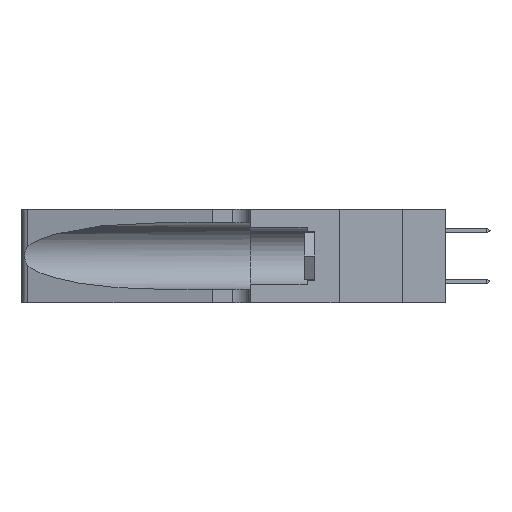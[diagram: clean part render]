
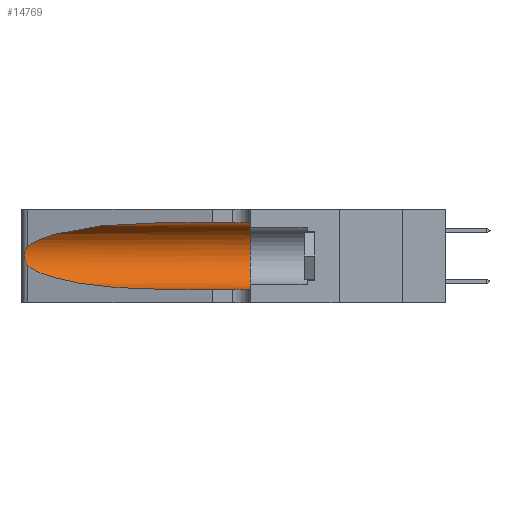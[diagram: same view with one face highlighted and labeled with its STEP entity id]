
A CAD part, left-side view. The second image highlights one B-rep face of the part: STEP entity #14769.
In plain terms, the highlighted cylindrical face has radius 3.308 mm (diameter 6.617 mm), a partial arc.
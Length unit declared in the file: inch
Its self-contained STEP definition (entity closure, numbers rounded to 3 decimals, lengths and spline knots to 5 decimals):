
#147 = CARTESIAN_POINT ( 'NONE',  ( 0.1305, 0.35, 0.185 ) ) ;
#178 = CARTESIAN_POINT ( 'NONE',  ( 0.25487, 1.22718, 0.14631 ) ) ;
#475 = CARTESIAN_POINT ( 'NONE',  ( 0.25555, 1.22994, 0.2215 ) ) ;
#570 = CARTESIAN_POINT ( 'NONE',  ( 0.25639, 1.23186, 0.15144 ) ) ;
#1190 = DIRECTION ( 'NONE',  ( 0., -1., 0. ) ) ;
#1701 = ORIENTED_EDGE ( 'NONE', *, *, #25862, .T. ) ;
#2406 = CARTESIAN_POINT ( 'NONE',  ( 0.2373, 1.15595, 0.08982 ) ) ;
#2423 = CARTESIAN_POINT ( 'NONE',  ( 0.1305, 0.35, 0.31525 ) ) ;
#2620 = DIRECTION ( 'NONE',  ( 0., 0., 1. ) ) ;
#3052 = CARTESIAN_POINT ( 'NONE',  ( 0.25487, 1.22718, 0.14631 ) ) ;
#3651 = CARTESIAN_POINT ( 'NONE',  ( 0.1305, 0.35, 0.05475 ) ) ;
#5392 = CARTESIAN_POINT ( 'NONE',  ( 0.25639, 1.23184, 0.21858 ) ) ;
#5688 = VECTOR ( 'NONE', #16708, 39.37008 ) ;
#5945 = CARTESIAN_POINT ( 'NONE',  ( 0.2373, 1.15595, 0.28018 ) ) ;
#5985 = DIRECTION ( 'NONE',  ( 0., 0., -1. ) ) ;
#6005 = CARTESIAN_POINT ( 'NONE',  ( 0.1305, 0.72297, 0.31525 ) ) ;
#6544 = EDGE_CURVE ( 'NONE', #20470, #12435, #19290, .T. ) ;
#6942 = ORIENTED_EDGE ( 'NONE', *, *, #23204, .T. ) ;
#7333 = CARTESIAN_POINT ( 'NONE',  ( 0.1305, 0.72297, 0.05475 ) ) ;
#7843 = ORIENTED_EDGE ( 'NONE', *, *, #6544, .T. ) ;
#7873 = CARTESIAN_POINT ( 'NONE',  ( 0.25854, 1.2359, 0.20912 ) ) ;
#9403 = ORIENTED_EDGE ( 'NONE', *, *, #28127, .T. ) ;
#9880 = CARTESIAN_POINT ( 'NONE',  ( 0.1305, 0.72297, 0.05475 ) ) ;
#10054 = VERTEX_POINT ( 'NONE', #2423 ) ;
#10321 = CARTESIAN_POINT ( 'NONE',  ( 0.26075, 1.23896, 0.19203 ) ) ;
#11560 = AXIS2_PLACEMENT_3D ( 'NONE', #147, #17246, #2620 ) ;
#12118 = CARTESIAN_POINT ( 'NONE',  ( 0.18966, 0.96281, 0.05475 ) ) ;
#12435 = VERTEX_POINT ( 'NONE', #9880 ) ;
#12780 = CARTESIAN_POINT ( 'NONE',  ( 0.26017, 1.23833, 0.17102 ) ) ;
#13754 = VECTOR ( 'NONE', #19162, 39.37008 ) ;
#14769 = ADVANCED_FACE ( 'NONE', ( #23942 ), #23166, .F. ) ;
#14770 = VERTEX_POINT ( 'NONE', #3651 ) ;
#15233 = CARTESIAN_POINT ( 'NONE',  ( 0.25789, 1.23486, 0.15765 ) ) ;
#15295 = CARTESIAN_POINT ( 'NONE',  ( 0.25487, 1.22718, 0.22369 ) ) ;
#15497 = EDGE_CURVE ( 'NONE', #10054, #14770, #21987, .T. ) ;
#15618 = AXIS2_PLACEMENT_3D ( 'NONE', #25443, #1190, #5985 ) ;
#15789 = VERTEX_POINT ( 'NONE', #6005 ) ;
#16371 = VERTEX_POINT ( 'NONE', #15295 ) ;
#16708 = DIRECTION ( 'NONE',  ( 0., -1., 0. ) ) ;
#17246 = DIRECTION ( 'NONE',  ( 0., 1., 0. ) ) ;
#17580 = CARTESIAN_POINT ( 'NONE',  ( 0.25487, 1.22718, 0.22369 ) ) ;
#17680 = CARTESIAN_POINT ( 'NONE',  ( 0.25555, 1.22993, 0.14849 ) ) ;
#19075 = EDGE_CURVE ( 'NONE', #15789, #10054, #30756, .T. ) ;
#19162 = DIRECTION ( 'NONE',  ( 0., -1., 0. ) ) ;
#19290 =( BOUNDED_CURVE ( )  B_SPLINE_CURVE ( 3, ( #21912, #2406, #12118, #7333 ),
 .UNSPECIFIED., .F., .T. ) 
 B_SPLINE_CURVE_WITH_KNOTS ( ( 4, 4 ),
 ( 3.44316, 4.71239 ),
 .UNSPECIFIED. ) 
 CURVE ( )  GEOMETRIC_REPRESENTATION_ITEM ( )  RATIONAL_B_SPLINE_CURVE ( ( 1., 0.87, 0.87, 1. ) ) 
 REPRESENTATION_ITEM ( '' )  );
#20219 = LINE ( 'NONE', #23930, #13754 ) ;
#20278 = B_SPLINE_CURVE_WITH_KNOTS ( 'NONE', 3,
 ( #17580, #475, #5392, #22435, #7873, #24867, #10321, #27282, #12780, #29732, #15233, #570, #17680, #3052 ),
 .UNSPECIFIED., .F., .F.,
 ( 4, 2, 2, 2, 2, 2, 4 ),
 ( 0., 0.00027, 0.00053, 0.00107, 0.0016, 0.00187, 0.00214 ),
 .UNSPECIFIED. ) ;
#20470 = VERTEX_POINT ( 'NONE', #178 ) ;
#20476 = CARTESIAN_POINT ( 'NONE',  ( 0.1305, 0.72297, 0.31525 ) ) ;
#21275 = ORIENTED_EDGE ( 'NONE', *, *, #15497, .F. ) ;
#21912 = CARTESIAN_POINT ( 'NONE',  ( 0.25487, 1.22718, 0.14631 ) ) ;
#21987 = CIRCLE ( 'NONE', #11560, 0.13025 ) ;
#22435 = CARTESIAN_POINT ( 'NONE',  ( 0.25787, 1.23484, 0.2124 ) ) ;
#22992 = CARTESIAN_POINT ( 'NONE',  ( 0.25487, 1.22718, 0.22369 ) ) ;
#23166 = CYLINDRICAL_SURFACE ( 'NONE', #15618, 0.13025 ) ;
#23204 = EDGE_CURVE ( 'NONE', #15789, #16371, #25861, .T. ) ;
#23930 = CARTESIAN_POINT ( 'NONE',  ( 0.1305, 1.61858, 0.05475 ) ) ;
#23942 = FACE_OUTER_BOUND ( 'NONE', #30150, .T. ) ;
#24867 = CARTESIAN_POINT ( 'NONE',  ( 0.26018, 1.23835, 0.19895 ) ) ;
#25303 = CARTESIAN_POINT ( 'NONE',  ( 0.18966, 0.96281, 0.31525 ) ) ;
#25443 = CARTESIAN_POINT ( 'NONE',  ( 0.1305, 1.61858, 0.185 ) ) ;
#25861 =( BOUNDED_CURVE ( )  B_SPLINE_CURVE ( 3, ( #20476, #25303, #5945, #22992 ),
 .UNSPECIFIED., .F., .T. ) 
 B_SPLINE_CURVE_WITH_KNOTS ( ( 4, 4 ),
 ( 1.5708, 2.84003 ),
 .UNSPECIFIED. ) 
 CURVE ( )  GEOMETRIC_REPRESENTATION_ITEM ( )  RATIONAL_B_SPLINE_CURVE ( ( 1., 0.87, 0.87, 1. ) ) 
 REPRESENTATION_ITEM ( '' )  );
#25862 = EDGE_CURVE ( 'NONE', #16371, #20470, #20278, .T. ) ;
#27282 = CARTESIAN_POINT ( 'NONE',  ( 0.26075, 1.23896, 0.178 ) ) ;
#28127 = EDGE_CURVE ( 'NONE', #12435, #14770, #20219, .T. ) ;
#29732 = CARTESIAN_POINT ( 'NONE',  ( 0.25856, 1.23593, 0.16098 ) ) ;
#30150 = EDGE_LOOP ( 'NONE', ( #6942, #1701, #7843, #9403, #21275, #30942 ) ) ;
#30756 = LINE ( 'NONE', #31175, #5688 ) ;
#30942 = ORIENTED_EDGE ( 'NONE', *, *, #19075, .F. ) ;
#31175 = CARTESIAN_POINT ( 'NONE',  ( 0.1305, 1.61858, 0.31525 ) ) ;
